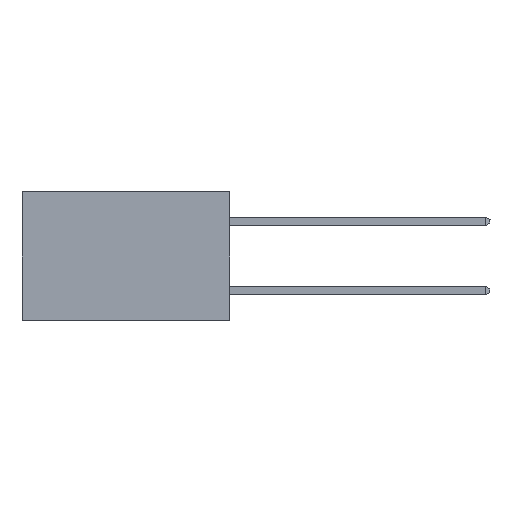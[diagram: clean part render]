
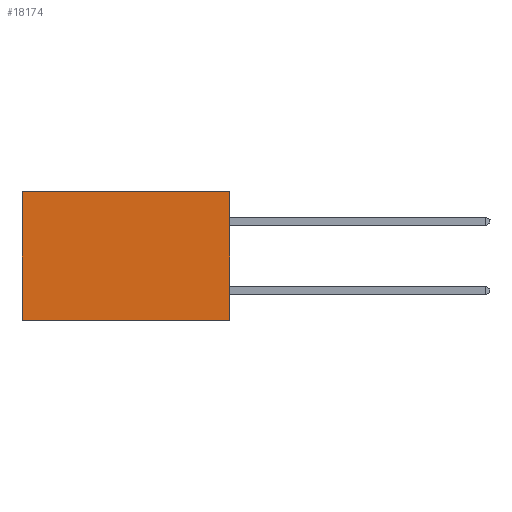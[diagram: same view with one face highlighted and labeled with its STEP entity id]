
A CAD part, left-side view. The second image highlights one B-rep face of the part: STEP entity #18174.
In plain terms, the highlighted planar face has unit normal (-1, 0, 0).
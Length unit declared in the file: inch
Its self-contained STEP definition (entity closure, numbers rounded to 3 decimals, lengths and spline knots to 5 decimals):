
#51 = DIRECTION ( 'NONE',  ( 0., 0., -1. ) ) ;
#146 = VECTOR ( 'NONE', #51, 39.37008 ) ;
#1365 = CARTESIAN_POINT ( 'NONE',  ( 0.2615, 0., 0. ) ) ;
#1809 = CARTESIAN_POINT ( 'NONE',  ( 0.2615, 0., -0.37 ) ) ;
#2298 = ORIENTED_EDGE ( 'NONE', *, *, #23087, .T. ) ;
#2875 = CARTESIAN_POINT ( 'NONE',  ( 0.2615, 0., -0.37 ) ) ;
#2982 = DIRECTION ( 'NONE',  ( 0., 0., -1. ) ) ;
#4293 = LINE ( 'NONE', #11198, #14961 ) ;
#4480 = LINE ( 'NONE', #22685, #9141 ) ;
#4863 = EDGE_CURVE ( 'NONE', #16933, #14982, #4480, .T. ) ;
#8006 = DIRECTION ( 'NONE',  ( 0., 1., 0. ) ) ;
#8580 = EDGE_CURVE ( 'NONE', #14982, #18618, #4293, .T. ) ;
#8828 = CARTESIAN_POINT ( 'NONE',  ( 0.2615, 0., 0. ) ) ;
#9141 = VECTOR ( 'NONE', #17511, 39.37008 ) ;
#9198 = LINE ( 'NONE', #18556, #146 ) ;
#9520 = EDGE_LOOP ( 'NONE', ( #12217, #22733, #16613, #2298 ) ) ;
#11198 = CARTESIAN_POINT ( 'NONE',  ( 0.2615, 0., -0.37 ) ) ;
#11359 = AXIS2_PLACEMENT_3D ( 'NONE', #2875, #11899, #2982 ) ;
#11899 = DIRECTION ( 'NONE',  ( 1., 0., 0. ) ) ;
#11970 = EDGE_CURVE ( 'NONE', #20859, #18618, #9198, .T. ) ;
#12217 = ORIENTED_EDGE ( 'NONE', *, *, #11970, .T. ) ;
#12752 = CARTESIAN_POINT ( 'NONE',  ( 0.2615, 0.6, 0. ) ) ;
#14227 = DIRECTION ( 'NONE',  ( 0., 1., 0. ) ) ;
#14961 = VECTOR ( 'NONE', #8006, 39.37008 ) ;
#14982 = VERTEX_POINT ( 'NONE', #1809 ) ;
#15672 = LINE ( 'NONE', #1365, #16581 ) ;
#16581 = VECTOR ( 'NONE', #14227, 39.37008 ) ;
#16613 = ORIENTED_EDGE ( 'NONE', *, *, #4863, .F. ) ;
#16933 = VERTEX_POINT ( 'NONE', #8828 ) ;
#17144 = CARTESIAN_POINT ( 'NONE',  ( 0.2615, 0.6, -0.37 ) ) ;
#17511 = DIRECTION ( 'NONE',  ( 0., 0., -1. ) ) ;
#18174 = ADVANCED_FACE ( 'NONE', ( #18923 ), #23054, .F. ) ;
#18556 = CARTESIAN_POINT ( 'NONE',  ( 0.2615, 0.6, -0.37 ) ) ;
#18618 = VERTEX_POINT ( 'NONE', #17144 ) ;
#18923 = FACE_OUTER_BOUND ( 'NONE', #9520, .T. ) ;
#20859 = VERTEX_POINT ( 'NONE', #12752 ) ;
#22685 = CARTESIAN_POINT ( 'NONE',  ( 0.2615, 0., -0.37 ) ) ;
#22733 = ORIENTED_EDGE ( 'NONE', *, *, #8580, .F. ) ;
#23054 = PLANE ( 'NONE',  #11359 ) ;
#23087 = EDGE_CURVE ( 'NONE', #16933, #20859, #15672, .T. ) ;
